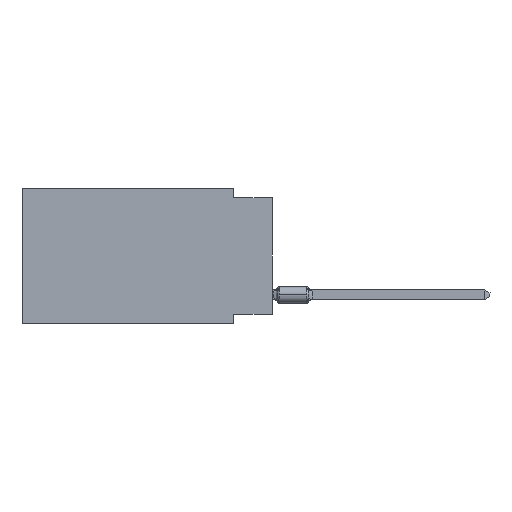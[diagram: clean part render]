
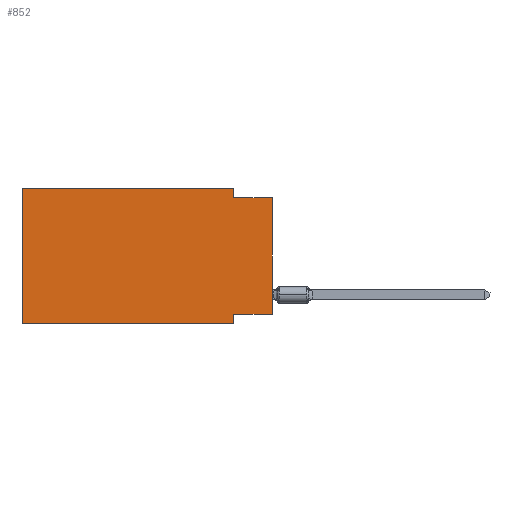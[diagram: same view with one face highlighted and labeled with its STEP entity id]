
A CAD part, left-side view. The second image highlights one B-rep face of the part: STEP entity #852.
In plain terms, the highlighted planar face has unit normal (-1, 0, 0).
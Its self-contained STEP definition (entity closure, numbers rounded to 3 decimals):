
#605 = VECTOR ( 'NONE', #23992, 1000. ) ;
#852 = ADVANCED_FACE ( 'NONE', ( #13278 ), #2335, .F. ) ;
#1057 = CARTESIAN_POINT ( 'NONE',  ( 0., 2.54, -0.635 ) ) ;
#1335 = VERTEX_POINT ( 'NONE', #22997 ) ;
#1954 = VECTOR ( 'NONE', #13547, 1000. ) ;
#2108 = EDGE_CURVE ( 'NONE', #18759, #23303, #13710, .T. ) ;
#2335 = PLANE ( 'NONE',  #19758 ) ;
#2405 = VECTOR ( 'NONE', #24049, 1000. ) ;
#2635 = LINE ( 'NONE', #11698, #18354 ) ;
#3061 = ORIENTED_EDGE ( 'NONE', *, *, #13526, .T. ) ;
#3611 = DIRECTION ( 'NONE',  ( 0., -1., 0. ) ) ;
#3657 = ORIENTED_EDGE ( 'NONE', *, *, #27019, .F. ) ;
#4561 = CARTESIAN_POINT ( 'NONE',  ( 0., 2.54, -8.89 ) ) ;
#4618 = LINE ( 'NONE', #13401, #2405 ) ;
#4908 = CARTESIAN_POINT ( 'NONE',  ( 0., 2.54, 0. ) ) ;
#6107 = ORIENTED_EDGE ( 'NONE', *, *, #12092, .T. ) ;
#7638 = VERTEX_POINT ( 'NONE', #17450 ) ;
#7647 = CARTESIAN_POINT ( 'NONE',  ( 0., 0., -8.255 ) ) ;
#8583 = ORIENTED_EDGE ( 'NONE', *, *, #12122, .F. ) ;
#8688 = ORIENTED_EDGE ( 'NONE', *, *, #2108, .F. ) ;
#8876 = VERTEX_POINT ( 'NONE', #27359 ) ;
#9234 = LINE ( 'NONE', #4908, #1954 ) ;
#9245 = VERTEX_POINT ( 'NONE', #16193 ) ;
#9681 = CARTESIAN_POINT ( 'NONE',  ( 0., 0., -8.255 ) ) ;
#11115 = CARTESIAN_POINT ( 'NONE',  ( 0., 16.383, 0. ) ) ;
#11698 = CARTESIAN_POINT ( 'NONE',  ( 0., 0., -0.635 ) ) ;
#12092 = EDGE_CURVE ( 'NONE', #18759, #7638, #12602, .T. ) ;
#12122 = EDGE_CURVE ( 'NONE', #1335, #19807, #4618, .T. ) ;
#12240 = LINE ( 'NONE', #13999, #26733 ) ;
#12602 = LINE ( 'NONE', #28215, #26298 ) ;
#12869 = EDGE_CURVE ( 'NONE', #19807, #23867, #9234, .T. ) ;
#13278 = FACE_OUTER_BOUND ( 'NONE', #18583, .T. ) ;
#13401 = CARTESIAN_POINT ( 'NONE',  ( 0., 16.383, 0. ) ) ;
#13526 = EDGE_CURVE ( 'NONE', #9245, #8876, #27095, .T. ) ;
#13547 = DIRECTION ( 'NONE',  ( 0., 0., -1. ) ) ;
#13710 = LINE ( 'NONE', #9681, #17994 ) ;
#13999 = CARTESIAN_POINT ( 'NONE',  ( 0., 16.383, 0. ) ) ;
#14225 = ORIENTED_EDGE ( 'NONE', *, *, #12869, .F. ) ;
#15086 = EDGE_CURVE ( 'NONE', #23867, #7638, #2635, .T. ) ;
#15745 = DIRECTION ( 'NONE',  ( 1., 0., 0. ) ) ;
#16193 = CARTESIAN_POINT ( 'NONE',  ( 0., 16.383, -8.89 ) ) ;
#17450 = CARTESIAN_POINT ( 'NONE',  ( 0., 0., -0.635 ) ) ;
#17994 = VECTOR ( 'NONE', #22786, 1000. ) ;
#18083 = EDGE_CURVE ( 'NONE', #9245, #1335, #12240, .T. ) ;
#18354 = VECTOR ( 'NONE', #20499, 1000. ) ;
#18583 = EDGE_LOOP ( 'NONE', ( #6107, #20182, #14225, #8583, #22871, #3061, #3657, #8688 ) ) ;
#18759 = VERTEX_POINT ( 'NONE', #7647 ) ;
#19304 = CARTESIAN_POINT ( 'NONE',  ( 0., 2.54, -8.255 ) ) ;
#19758 = AXIS2_PLACEMENT_3D ( 'NONE', #11115, #15745, #19910 ) ;
#19807 = VERTEX_POINT ( 'NONE', #26975 ) ;
#19910 = DIRECTION ( 'NONE',  ( 0., 0., -1. ) ) ;
#20182 = ORIENTED_EDGE ( 'NONE', *, *, #15086, .F. ) ;
#20499 = DIRECTION ( 'NONE',  ( 0., -1., 0. ) ) ;
#20908 = DIRECTION ( 'NONE',  ( 0., 0., 1. ) ) ;
#21476 = VECTOR ( 'NONE', #3611, 1000. ) ;
#22051 = DIRECTION ( 'NONE',  ( 0., 0., 1. ) ) ;
#22786 = DIRECTION ( 'NONE',  ( 0., 1., 0. ) ) ;
#22871 = ORIENTED_EDGE ( 'NONE', *, *, #18083, .F. ) ;
#22997 = CARTESIAN_POINT ( 'NONE',  ( 0., 16.383, 0. ) ) ;
#23303 = VERTEX_POINT ( 'NONE', #19304 ) ;
#23338 = CARTESIAN_POINT ( 'NONE',  ( 0., 16.383, -8.89 ) ) ;
#23867 = VERTEX_POINT ( 'NONE', #1057 ) ;
#23992 = DIRECTION ( 'NONE',  ( 0., 0., -1. ) ) ;
#24049 = DIRECTION ( 'NONE',  ( 0., -1., 0. ) ) ;
#24577 = LINE ( 'NONE', #4561, #605 ) ;
#26298 = VECTOR ( 'NONE', #22051, 1000. ) ;
#26733 = VECTOR ( 'NONE', #20908, 1000. ) ;
#26975 = CARTESIAN_POINT ( 'NONE',  ( 0., 2.54, 0. ) ) ;
#27019 = EDGE_CURVE ( 'NONE', #23303, #8876, #24577, .T. ) ;
#27095 = LINE ( 'NONE', #23338, #21476 ) ;
#27359 = CARTESIAN_POINT ( 'NONE',  ( 0., 2.54, -8.89 ) ) ;
#28215 = CARTESIAN_POINT ( 'NONE',  ( 0., 0., 0. ) ) ;
